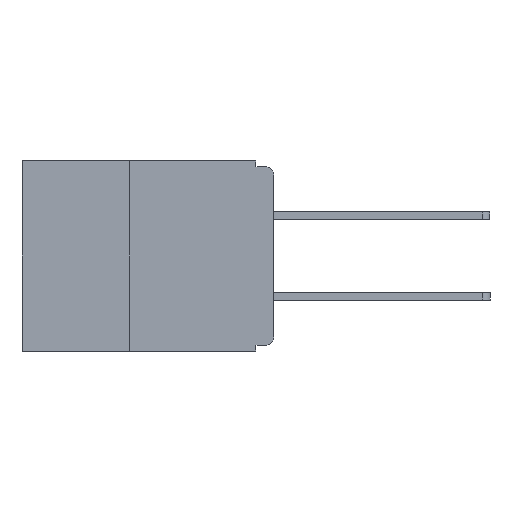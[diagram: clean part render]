
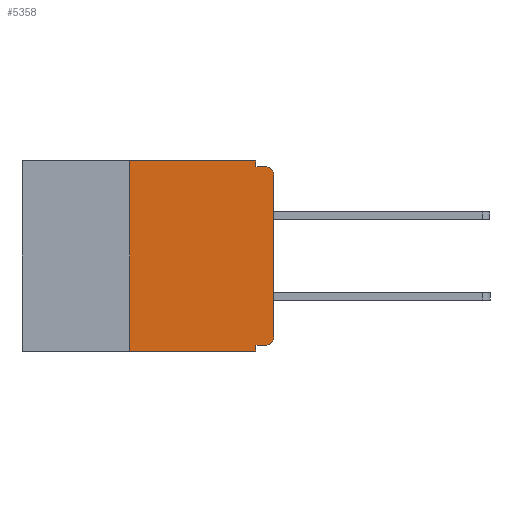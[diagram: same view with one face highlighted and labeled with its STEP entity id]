
A CAD part, left-side view. The second image highlights one B-rep face of the part: STEP entity #5358.
In plain terms, the highlighted planar face has unit normal (-1, 0, 0).
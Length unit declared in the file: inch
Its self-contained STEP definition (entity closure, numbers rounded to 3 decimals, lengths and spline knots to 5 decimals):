
#473 = CARTESIAN_POINT ( 'NONE',  ( 0., 0., -0.32 ) ) ;
#582 = EDGE_CURVE ( 'NONE', #15579, #18606, #4993, .T. ) ;
#935 = CARTESIAN_POINT ( 'NONE',  ( 0., 0.25, -0.33 ) ) ;
#1341 = DIRECTION ( 'NONE',  ( 0., -1., 0. ) ) ;
#1342 = VERTEX_POINT ( 'NONE', #3375 ) ;
#2028 = DIRECTION ( 'NONE',  ( -1., 0., 0. ) ) ;
#2060 = DIRECTION ( 'NONE',  ( 0., 0., -1. ) ) ;
#2301 = DIRECTION ( 'NONE',  ( 0., 0., 1. ) ) ;
#2323 = CARTESIAN_POINT ( 'NONE',  ( 0., 0.25, -0.33 ) ) ;
#3040 = DIRECTION ( 'NONE',  ( 0., 0., -1. ) ) ;
#3105 = CARTESIAN_POINT ( 'NONE',  ( 0., 0., -0.01 ) ) ;
#3375 = CARTESIAN_POINT ( 'NONE',  ( 0., 0.031, 0. ) ) ;
#3578 = CARTESIAN_POINT ( 'NONE',  ( 0., 0., 0. ) ) ;
#3732 = AXIS2_PLACEMENT_3D ( 'NONE', #14743, #14721, #14708 ) ;
#3763 = CARTESIAN_POINT ( 'NONE',  ( 0., 0.031, -0.01 ) ) ;
#3765 = LINE ( 'NONE', #12199, #14874 ) ;
#3833 = VECTOR ( 'NONE', #1341, 39.37008 ) ;
#4783 = EDGE_CURVE ( 'NONE', #10270, #6259, #19566, .T. ) ;
#4993 = LINE ( 'NONE', #3105, #12083 ) ;
#5198 = EDGE_CURVE ( 'NONE', #16679, #18606, #19508, .T. ) ;
#5263 = FACE_OUTER_BOUND ( 'NONE', #16267, .T. ) ;
#5358 = ADVANCED_FACE ( 'NONE', ( #5263 ), #14978, .F. ) ;
#5507 = CARTESIAN_POINT ( 'NONE',  ( 0., 0.031, -0.32 ) ) ;
#5767 = CARTESIAN_POINT ( 'NONE',  ( 0., 0.25, 0. ) ) ;
#5843 = DIRECTION ( 'NONE',  ( 0., -1., 0. ) ) ;
#5926 = AXIS2_PLACEMENT_3D ( 'NONE', #11189, #2028, #12682 ) ;
#6203 = EDGE_CURVE ( 'NONE', #6259, #1342, #10220, .T. ) ;
#6257 = DIRECTION ( 'NONE',  ( 0., -1., 0. ) ) ;
#6259 = VERTEX_POINT ( 'NONE', #5767 ) ;
#6277 = VERTEX_POINT ( 'NONE', #5507 ) ;
#6353 = CARTESIAN_POINT ( 'NONE',  ( 0., 0.437, 0. ) ) ;
#6870 = EDGE_CURVE ( 'NONE', #1342, #15579, #3765, .T. ) ;
#6937 = CIRCLE ( 'NONE', #5926, 0.015 ) ;
#8292 = EDGE_CURVE ( 'NONE', #16832, #6277, #9438, .T. ) ;
#8526 = LINE ( 'NONE', #3578, #16476 ) ;
#8965 = VECTOR ( 'NONE', #9735, 39.37008 ) ;
#8971 = CARTESIAN_POINT ( 'NONE',  ( 0., 0., -0.305 ) ) ;
#9438 = LINE ( 'NONE', #473, #8965 ) ;
#9735 = DIRECTION ( 'NONE',  ( 0., 1., 0. ) ) ;
#10220 = LINE ( 'NONE', #6353, #18597 ) ;
#10233 = AXIS2_PLACEMENT_3D ( 'NONE', #16346, #16323, #16302 ) ;
#10270 = VERTEX_POINT ( 'NONE', #935 ) ;
#11189 = CARTESIAN_POINT ( 'NONE',  ( 0., 0.015, -0.305 ) ) ;
#11579 = CARTESIAN_POINT ( 'NONE',  ( 0., 0.031, -0.33 ) ) ;
#11721 = VECTOR ( 'NONE', #2301, 39.37008 ) ;
#11813 = CARTESIAN_POINT ( 'NONE',  ( 0., 0.015, -0.01 ) ) ;
#12024 = ORIENTED_EDGE ( 'NONE', *, *, #13909, .T. ) ;
#12041 = ORIENTED_EDGE ( 'NONE', *, *, #5198, .T. ) ;
#12083 = VECTOR ( 'NONE', #5843, 39.37008 ) ;
#12199 = CARTESIAN_POINT ( 'NONE',  ( 0., 0.031, 0. ) ) ;
#12362 = ORIENTED_EDGE ( 'NONE', *, *, #582, .F. ) ;
#12495 = ORIENTED_EDGE ( 'NONE', *, *, #6870, .F. ) ;
#12530 = ORIENTED_EDGE ( 'NONE', *, *, #6203, .F. ) ;
#12554 = ORIENTED_EDGE ( 'NONE', *, *, #4783, .F. ) ;
#12640 = ORIENTED_EDGE ( 'NONE', *, *, #18242, .T. ) ;
#12650 = DIRECTION ( 'NONE',  ( 0., 0., 1. ) ) ;
#12682 = DIRECTION ( 'NONE',  ( 0., 0., -1. ) ) ;
#12728 = ORIENTED_EDGE ( 'NONE', *, *, #17270, .F. ) ;
#12867 = VERTEX_POINT ( 'NONE', #11579 ) ;
#12879 = ORIENTED_EDGE ( 'NONE', *, *, #8292, .F. ) ;
#13010 = ORIENTED_EDGE ( 'NONE', *, *, #19562, .T. ) ;
#13909 = EDGE_CURVE ( 'NONE', #19299, #16679, #8526, .T. ) ;
#14290 = VECTOR ( 'NONE', #2060, 39.37008 ) ;
#14708 = DIRECTION ( 'NONE',  ( 0., 0., -1. ) ) ;
#14721 = DIRECTION ( 'NONE',  ( 1., 0., 0. ) ) ;
#14743 = CARTESIAN_POINT ( 'NONE',  ( 0., 0.437, 0. ) ) ;
#14874 = VECTOR ( 'NONE', #3040, 39.37008 ) ;
#14978 = PLANE ( 'NONE',  #3732 ) ;
#15579 = VERTEX_POINT ( 'NONE', #3763 ) ;
#15877 = LINE ( 'NONE', #19377, #3833 ) ;
#16267 = EDGE_LOOP ( 'NONE', ( #12024, #12041, #12362, #12495, #12530, #12554, #12640, #12728, #12879, #13010 ) ) ;
#16302 = DIRECTION ( 'NONE',  ( 0., 0., -1. ) ) ;
#16323 = DIRECTION ( 'NONE',  ( -1., 0., 0. ) ) ;
#16346 = CARTESIAN_POINT ( 'NONE',  ( 0., 0.015, -0.025 ) ) ;
#16476 = VECTOR ( 'NONE', #12650, 39.37008 ) ;
#16679 = VERTEX_POINT ( 'NONE', #17124 ) ;
#16832 = VERTEX_POINT ( 'NONE', #18999 ) ;
#17124 = CARTESIAN_POINT ( 'NONE',  ( 0., 0., -0.025 ) ) ;
#17165 = CARTESIAN_POINT ( 'NONE',  ( 0., 0.031, -0.33 ) ) ;
#17270 = EDGE_CURVE ( 'NONE', #6277, #12867, #18234, .T. ) ;
#18234 = LINE ( 'NONE', #17165, #14290 ) ;
#18242 = EDGE_CURVE ( 'NONE', #10270, #12867, #15877, .T. ) ;
#18597 = VECTOR ( 'NONE', #6257, 39.37008 ) ;
#18606 = VERTEX_POINT ( 'NONE', #11813 ) ;
#18999 = CARTESIAN_POINT ( 'NONE',  ( 0., 0.015, -0.32 ) ) ;
#19299 = VERTEX_POINT ( 'NONE', #8971 ) ;
#19377 = CARTESIAN_POINT ( 'NONE',  ( 0., 0.437, -0.33 ) ) ;
#19508 = CIRCLE ( 'NONE', #10233, 0.015 ) ;
#19562 = EDGE_CURVE ( 'NONE', #16832, #19299, #6937, .T. ) ;
#19566 = LINE ( 'NONE', #2323, #11721 ) ;
